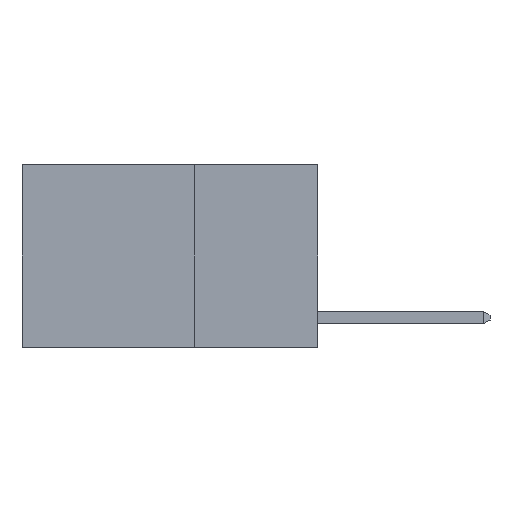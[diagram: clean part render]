
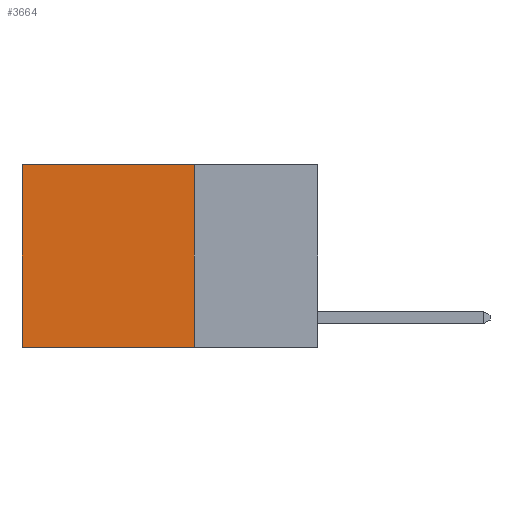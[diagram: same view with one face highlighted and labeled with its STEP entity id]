
A CAD part, left-side view. The second image highlights one B-rep face of the part: STEP entity #3664.
In plain terms, the highlighted planar face has unit normal (-1, 0, 0).
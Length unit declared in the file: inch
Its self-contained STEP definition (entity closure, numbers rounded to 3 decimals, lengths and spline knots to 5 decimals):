
#5 = CARTESIAN_POINT ( 'NONE',  ( 0.2625, 0.25, 0. ) ) ;
#38 = EDGE_CURVE ( 'NONE', #9293, #6807, #1829, .T. ) ;
#150 = CARTESIAN_POINT ( 'NONE',  ( 0.2625, 0.25, 0. ) ) ;
#391 = LINE ( 'NONE', #4087, #8640 ) ;
#962 = DIRECTION ( 'NONE',  ( 0., 0., -1. ) ) ;
#1214 = VECTOR ( 'NONE', #8813, 39.37008 ) ;
#1563 = CARTESIAN_POINT ( 'NONE',  ( 0.2625, 0.25, -0.37 ) ) ;
#1621 = ORIENTED_EDGE ( 'NONE', *, *, #38, .F. ) ;
#1829 = LINE ( 'NONE', #5, #10236 ) ;
#1883 = ORIENTED_EDGE ( 'NONE', *, *, #2130, .T. ) ;
#2130 = EDGE_CURVE ( 'NONE', #9293, #3643, #8851, .T. ) ;
#2764 = CARTESIAN_POINT ( 'NONE',  ( 0.2625, 0.6, -0.37 ) ) ;
#2799 = VECTOR ( 'NONE', #10274, 39.37008 ) ;
#3081 = CARTESIAN_POINT ( 'NONE',  ( 0.2625, 0.6, 0. ) ) ;
#3156 = LINE ( 'NONE', #3081, #1214 ) ;
#3305 = EDGE_CURVE ( 'NONE', #3643, #9652, #3156, .T. ) ;
#3643 = VERTEX_POINT ( 'NONE', #6800 ) ;
#3664 = ADVANCED_FACE ( 'NONE', ( #6711 ), #8384, .F. ) ;
#4087 = CARTESIAN_POINT ( 'NONE',  ( 0.2625, 0.25, -0.37 ) ) ;
#4435 = EDGE_LOOP ( 'NONE', ( #5842, #7988, #1621, #1883 ) ) ;
#5842 = ORIENTED_EDGE ( 'NONE', *, *, #3305, .T. ) ;
#6007 = DIRECTION ( 'NONE',  ( 1., 0., 0. ) ) ;
#6138 = EDGE_CURVE ( 'NONE', #6807, #9652, #391, .T. ) ;
#6711 = FACE_OUTER_BOUND ( 'NONE', #4435, .T. ) ;
#6800 = CARTESIAN_POINT ( 'NONE',  ( 0.2625, 0.6, 0. ) ) ;
#6807 = VERTEX_POINT ( 'NONE', #1563 ) ;
#7988 = ORIENTED_EDGE ( 'NONE', *, *, #6138, .F. ) ;
#8051 = CARTESIAN_POINT ( 'NONE',  ( 0.2625, 0.25, 0. ) ) ;
#8384 = PLANE ( 'NONE',  #8480 ) ;
#8480 = AXIS2_PLACEMENT_3D ( 'NONE', #150, #6007, #962 ) ;
#8625 = DIRECTION ( 'NONE',  ( 0., 0., -1. ) ) ;
#8640 = VECTOR ( 'NONE', #8946, 39.37008 ) ;
#8747 = CARTESIAN_POINT ( 'NONE',  ( 0.2625, 0.25, 0. ) ) ;
#8813 = DIRECTION ( 'NONE',  ( 0., 0., -1. ) ) ;
#8851 = LINE ( 'NONE', #8747, #2799 ) ;
#8946 = DIRECTION ( 'NONE',  ( 0., 1., 0. ) ) ;
#9293 = VERTEX_POINT ( 'NONE', #8051 ) ;
#9652 = VERTEX_POINT ( 'NONE', #2764 ) ;
#10236 = VECTOR ( 'NONE', #8625, 39.37008 ) ;
#10274 = DIRECTION ( 'NONE',  ( 0., 1., 0. ) ) ;
